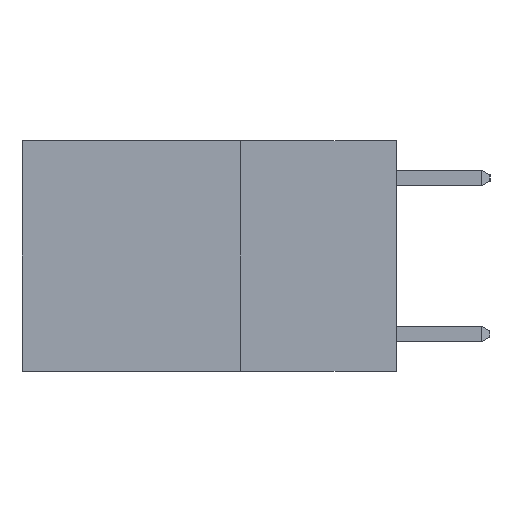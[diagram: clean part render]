
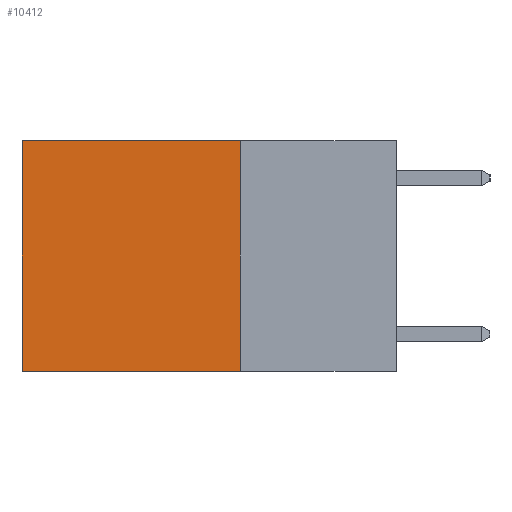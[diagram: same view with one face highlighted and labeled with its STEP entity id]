
A CAD part, left-side view. The second image highlights one B-rep face of the part: STEP entity #10412.
In plain terms, the highlighted planar face has unit normal (-1, 0, 0).
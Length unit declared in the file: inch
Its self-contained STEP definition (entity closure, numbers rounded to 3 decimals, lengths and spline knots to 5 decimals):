
#321 = AXIS2_PLACEMENT_3D ( 'NONE', #10019, #8249, #2427 ) ;
#403 = EDGE_CURVE ( 'NONE', #3562, #10980, #6299, .T. ) ;
#836 = CARTESIAN_POINT ( 'NONE',  ( 0.2625, 0.25, -0.37 ) ) ;
#1405 = DIRECTION ( 'NONE',  ( 0., 0., -1. ) ) ;
#1561 = CARTESIAN_POINT ( 'NONE',  ( 0.2625, 0.25, -0.37 ) ) ;
#1708 = CARTESIAN_POINT ( 'NONE',  ( 0.2625, 0.25, 0. ) ) ;
#1854 = FACE_OUTER_BOUND ( 'NONE', #10720, .T. ) ;
#2190 = VERTEX_POINT ( 'NONE', #5566 ) ;
#2394 = CARTESIAN_POINT ( 'NONE',  ( 0.2625, 0.6, 0. ) ) ;
#2427 = DIRECTION ( 'NONE',  ( 0., 0., -1. ) ) ;
#2539 = CARTESIAN_POINT ( 'NONE',  ( 0.2625, 0.6, 0. ) ) ;
#3562 = VERTEX_POINT ( 'NONE', #1561 ) ;
#4725 = DIRECTION ( 'NONE',  ( 0., 1., 0. ) ) ;
#5113 = ORIENTED_EDGE ( 'NONE', *, *, #9462, .T. ) ;
#5401 = PLANE ( 'NONE',  #321 ) ;
#5566 = CARTESIAN_POINT ( 'NONE',  ( 0.2625, 0.25, 0. ) ) ;
#5628 = DIRECTION ( 'NONE',  ( 0., 0., -1. ) ) ;
#6299 = LINE ( 'NONE', #836, #10850 ) ;
#6416 = VECTOR ( 'NONE', #4725, 39.37008 ) ;
#6684 = LINE ( 'NONE', #2394, #12060 ) ;
#6763 = DIRECTION ( 'NONE',  ( 0., 1., 0. ) ) ;
#7546 = VERTEX_POINT ( 'NONE', #2539 ) ;
#7690 = LINE ( 'NONE', #9335, #12186 ) ;
#8113 = CARTESIAN_POINT ( 'NONE',  ( 0.2625, 0.6, -0.37 ) ) ;
#8249 = DIRECTION ( 'NONE',  ( 1., 0., 0. ) ) ;
#8528 = ORIENTED_EDGE ( 'NONE', *, *, #403, .F. ) ;
#8548 = LINE ( 'NONE', #1708, #6416 ) ;
#9056 = ORIENTED_EDGE ( 'NONE', *, *, #9992, .F. ) ;
#9335 = CARTESIAN_POINT ( 'NONE',  ( 0.2625, 0.25, 0. ) ) ;
#9462 = EDGE_CURVE ( 'NONE', #2190, #7546, #8548, .T. ) ;
#9518 = ORIENTED_EDGE ( 'NONE', *, *, #9840, .T. ) ;
#9840 = EDGE_CURVE ( 'NONE', #7546, #10980, #6684, .T. ) ;
#9992 = EDGE_CURVE ( 'NONE', #2190, #3562, #7690, .T. ) ;
#10019 = CARTESIAN_POINT ( 'NONE',  ( 0.2625, 0.25, 0. ) ) ;
#10412 = ADVANCED_FACE ( 'NONE', ( #1854 ), #5401, .F. ) ;
#10720 = EDGE_LOOP ( 'NONE', ( #9518, #8528, #9056, #5113 ) ) ;
#10850 = VECTOR ( 'NONE', #6763, 39.37008 ) ;
#10980 = VERTEX_POINT ( 'NONE', #8113 ) ;
#12060 = VECTOR ( 'NONE', #1405, 39.37008 ) ;
#12186 = VECTOR ( 'NONE', #5628, 39.37008 ) ;
